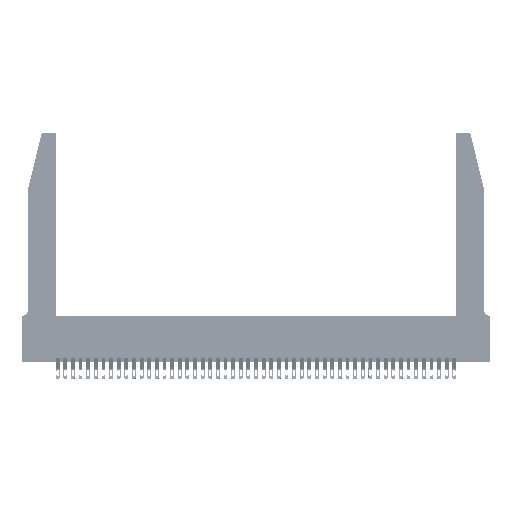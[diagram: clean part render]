
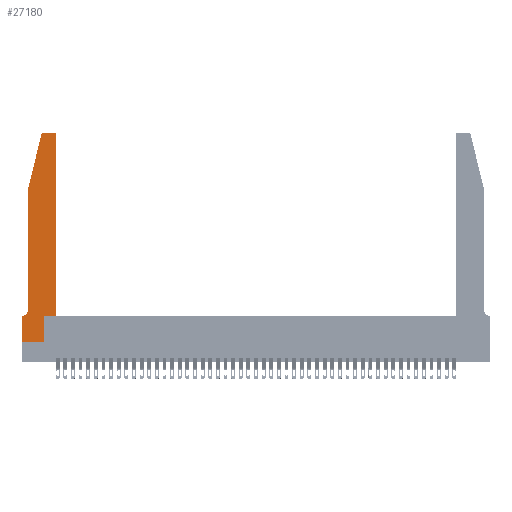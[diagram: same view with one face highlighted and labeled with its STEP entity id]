
A CAD part, top view. The second image highlights one B-rep face of the part: STEP entity #27180.
In plain terms, the highlighted planar face has unit normal (0, 0, 1).
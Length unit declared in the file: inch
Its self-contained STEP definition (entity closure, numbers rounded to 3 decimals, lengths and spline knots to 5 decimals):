
#801 = ORIENTED_EDGE ( 'NONE', *, *, #11552, .T. ) ;
#1193 = CARTESIAN_POINT ( 'NONE',  ( 0.284, 2.72, 0.37 ) ) ;
#1304 = EDGE_CURVE ( 'NONE', #40072, #29603, #14890, .T. ) ;
#1681 = FACE_OUTER_BOUND ( 'NONE', #29693, .T. ) ;
#1839 = LINE ( 'NONE', #11307, #22044 ) ;
#2022 = ORIENTED_EDGE ( 'NONE', *, *, #25319, .T. ) ;
#2375 = ORIENTED_EDGE ( 'NONE', *, *, #26053, .T. ) ;
#2420 = VERTEX_POINT ( 'NONE', #45170 ) ;
#2637 = DIRECTION ( 'NONE',  ( 1., 0., 0. ) ) ;
#2757 = CARTESIAN_POINT ( 'NONE',  ( 0.4205, 2.75, 0.37 ) ) ;
#3232 = VECTOR ( 'NONE', #33216, 39.37008 ) ;
#3350 = AXIS2_PLACEMENT_3D ( 'NONE', #37500, #37949, #27576 ) ;
#4130 = EDGE_CURVE ( 'NONE', #29603, #31994, #12475, .T. ) ;
#4559 = AXIS2_PLACEMENT_3D ( 'NONE', #44286, #23397, #6246 ) ;
#4646 = CARTESIAN_POINT ( 'NONE',  ( 0.2865, 0.35, 0.37 ) ) ;
#4912 = DIRECTION ( 'NONE',  ( 0., 0., 1. ) ) ;
#6246 = DIRECTION ( 'NONE',  ( -1., 0., 0. ) ) ;
#6856 = EDGE_CURVE ( 'NONE', #2420, #23568, #24761, .T. ) ;
#7290 = DIRECTION ( 'NONE',  ( -1., 0., 0. ) ) ;
#8153 = ORIENTED_EDGE ( 'NONE', *, *, #1304, .T. ) ;
#9876 = DIRECTION ( 'NONE',  ( 1., 0., 0. ) ) ;
#10020 = DIRECTION ( 'NONE',  ( -1., 0., 0. ) ) ;
#10083 = VERTEX_POINT ( 'NONE', #37987 ) ;
#10771 = VECTOR ( 'NONE', #10020, 39.37008 ) ;
#11307 = CARTESIAN_POINT ( 'NONE',  ( 0.0755, 0.35, 0.37 ) ) ;
#11552 = EDGE_CURVE ( 'NONE', #24184, #2420, #42702, .T. ) ;
#12133 = VECTOR ( 'NONE', #22312, 39.37008 ) ;
#12475 = LINE ( 'NONE', #16951, #10771 ) ;
#12736 = VERTEX_POINT ( 'NONE', #39679 ) ;
#12851 = DIRECTION ( 'NONE',  ( 0., -1., 0. ) ) ;
#12891 = VERTEX_POINT ( 'NONE', #44374 ) ;
#13064 = VECTOR ( 'NONE', #12851, 39.37008 ) ;
#14890 = CIRCLE ( 'NONE', #3350, 0.03 ) ;
#15412 = CARTESIAN_POINT ( 'NONE',  ( 0.2865, 0., 0.37 ) ) ;
#16541 = CARTESIAN_POINT ( 'NONE',  ( 0.0755, 2., 0.37 ) ) ;
#16951 = CARTESIAN_POINT ( 'NONE',  ( 0.2605, 2.75, 0.37 ) ) ;
#18939 = VECTOR ( 'NONE', #27300, 39.37008 ) ;
#19189 = DIRECTION ( 'NONE',  ( 1., 0., 0. ) ) ;
#19349 = CARTESIAN_POINT ( 'NONE',  ( 0., 0., 0.37 ) ) ;
#20262 = EDGE_CURVE ( 'NONE', #28550, #41834, #31732, .T. ) ;
#20722 = PLANE ( 'NONE',  #41174 ) ;
#21221 = LINE ( 'NONE', #16541, #13064 ) ;
#21244 = CARTESIAN_POINT ( 'NONE',  ( 0.4505, 0.35, 0.37 ) ) ;
#21932 = EDGE_CURVE ( 'NONE', #10083, #44699, #31097, .T. ) ;
#22044 = VECTOR ( 'NONE', #7290, 39.37008 ) ;
#22248 = ORIENTED_EDGE ( 'NONE', *, *, #27898, .T. ) ;
#22312 = DIRECTION ( 'NONE',  ( 1., 0., 0. ) ) ;
#23012 = ORIENTED_EDGE ( 'NONE', *, *, #20262, .T. ) ;
#23226 = CARTESIAN_POINT ( 'NONE',  ( 0.4505, 2.72, 0.37 ) ) ;
#23397 = DIRECTION ( 'NONE',  ( 0., 0., -1. ) ) ;
#23568 = VERTEX_POINT ( 'NONE', #15412 ) ;
#24109 = EDGE_CURVE ( 'NONE', #23568, #28550, #28151, .T. ) ;
#24184 = VERTEX_POINT ( 'NONE', #34735 ) ;
#24550 = CARTESIAN_POINT ( 'NONE',  ( 0.0755, 2., 0.37 ) ) ;
#24761 = LINE ( 'NONE', #44506, #44985 ) ;
#24845 = ORIENTED_EDGE ( 'NONE', *, *, #6856, .T. ) ;
#24853 = DIRECTION ( 'NONE',  ( 0., 1., 0. ) ) ;
#25319 = EDGE_CURVE ( 'NONE', #12891, #12736, #39002, .T. ) ;
#26053 = EDGE_CURVE ( 'NONE', #12736, #24184, #1839, .T. ) ;
#26388 = ORIENTED_EDGE ( 'NONE', *, *, #21932, .T. ) ;
#26883 = CARTESIAN_POINT ( 'NONE',  ( 0.0755, 2., 0.37 ) ) ;
#27180 = ADVANCED_FACE ( 'NONE', ( #1681 ), #20722, .T. ) ;
#27300 = DIRECTION ( 'NONE',  ( 0., 1., 0. ) ) ;
#27576 = DIRECTION ( 'NONE',  ( 1., 0., 0. ) ) ;
#27898 = EDGE_CURVE ( 'NONE', #41834, #40072, #39834, .T. ) ;
#28151 = LINE ( 'NONE', #37376, #18939 ) ;
#28210 = DIRECTION ( 'NONE',  ( 0., -1., 0. ) ) ;
#28550 = VERTEX_POINT ( 'NONE', #4646 ) ;
#29258 = EDGE_CURVE ( 'NONE', #31994, #10083, #42423, .T. ) ;
#29603 = VERTEX_POINT ( 'NONE', #2757 ) ;
#29693 = EDGE_LOOP ( 'NONE', ( #33811, #35302, #26388, #41984, #2022, #2375, #801, #24845, #37142, #23012, #22248, #8153 ) ) ;
#29798 = CARTESIAN_POINT ( 'NONE',  ( 0.4505, 0.35, 0.37 ) ) ;
#31097 = LINE ( 'NONE', #24550, #3232 ) ;
#31732 = LINE ( 'NONE', #29798, #12133 ) ;
#31994 = VERTEX_POINT ( 'NONE', #45202 ) ;
#33216 = DIRECTION ( 'NONE',  ( -0.239, -0.971, 0. ) ) ;
#33811 = ORIENTED_EDGE ( 'NONE', *, *, #4130, .T. ) ;
#34735 = CARTESIAN_POINT ( 'NONE',  ( 0., 0.35, 0.37 ) ) ;
#35302 = ORIENTED_EDGE ( 'NONE', *, *, #29258, .T. ) ;
#37142 = ORIENTED_EDGE ( 'NONE', *, *, #24109, .T. ) ;
#37376 = CARTESIAN_POINT ( 'NONE',  ( 0.2865, 0.35, 0.37 ) ) ;
#37500 = CARTESIAN_POINT ( 'NONE',  ( 0.4205, 2.72, 0.37 ) ) ;
#37949 = DIRECTION ( 'NONE',  ( 0., 0., 1. ) ) ;
#37987 = CARTESIAN_POINT ( 'NONE',  ( 0.25487, 2.72718, 0.37 ) ) ;
#38369 = VECTOR ( 'NONE', #28210, 39.37008 ) ;
#38906 = EDGE_CURVE ( 'NONE', #44699, #12891, #21221, .T. ) ;
#39002 = CIRCLE ( 'NONE', #4559, 0.07 ) ;
#39679 = CARTESIAN_POINT ( 'NONE',  ( 0.0055, 0.35, 0.37 ) ) ;
#39834 = LINE ( 'NONE', #44906, #42033 ) ;
#40072 = VERTEX_POINT ( 'NONE', #23226 ) ;
#41174 = AXIS2_PLACEMENT_3D ( 'NONE', #44522, #45099, #9876 ) ;
#41834 = VERTEX_POINT ( 'NONE', #21244 ) ;
#41984 = ORIENTED_EDGE ( 'NONE', *, *, #38906, .T. ) ;
#42033 = VECTOR ( 'NONE', #24853, 39.37008 ) ;
#42423 = CIRCLE ( 'NONE', #44220, 0.03 ) ;
#42702 = LINE ( 'NONE', #19349, #38369 ) ;
#44220 = AXIS2_PLACEMENT_3D ( 'NONE', #1193, #4912, #19189 ) ;
#44286 = CARTESIAN_POINT ( 'NONE',  ( 0.0055, 0.42, 0.37 ) ) ;
#44374 = CARTESIAN_POINT ( 'NONE',  ( 0.0755, 0.42, 0.37 ) ) ;
#44506 = CARTESIAN_POINT ( 'NONE',  ( 0., 0., 0.37 ) ) ;
#44522 = CARTESIAN_POINT ( 'NONE',  ( 0., 0.35, 0.37 ) ) ;
#44699 = VERTEX_POINT ( 'NONE', #26883 ) ;
#44906 = CARTESIAN_POINT ( 'NONE',  ( 0.4505, 0.35, 0.37 ) ) ;
#44985 = VECTOR ( 'NONE', #2637, 39.37008 ) ;
#45099 = DIRECTION ( 'NONE',  ( 0., 0., 1. ) ) ;
#45170 = CARTESIAN_POINT ( 'NONE',  ( 0., 0., 0.37 ) ) ;
#45202 = CARTESIAN_POINT ( 'NONE',  ( 0.284, 2.75, 0.37 ) ) ;
